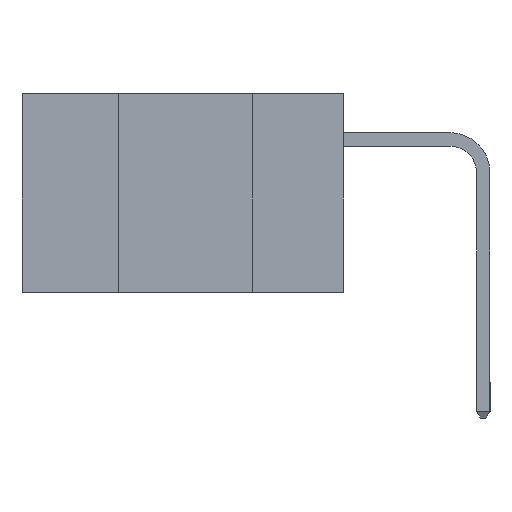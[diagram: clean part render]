
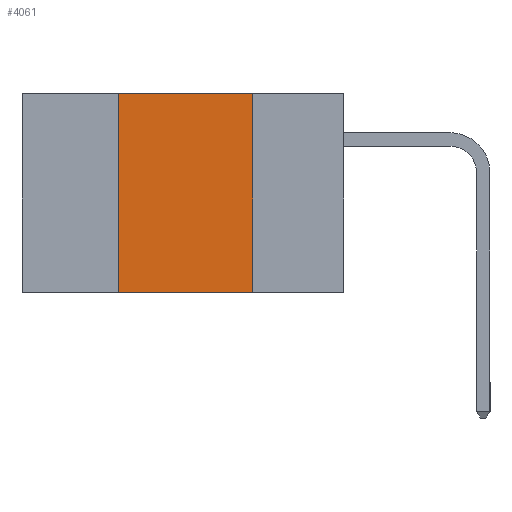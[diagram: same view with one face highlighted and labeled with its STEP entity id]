
A CAD part, left-side view. The second image highlights one B-rep face of the part: STEP entity #4061.
In plain terms, the highlighted planar face has unit normal (-1, 0, 0).
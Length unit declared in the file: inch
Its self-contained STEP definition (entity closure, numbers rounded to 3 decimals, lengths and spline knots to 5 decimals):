
#245 = CARTESIAN_POINT ( 'NONE',  ( 0., 0.17, -0.37 ) ) ;
#361 = CARTESIAN_POINT ( 'NONE',  ( 0., 0.6, -0.37 ) ) ;
#734 = CARTESIAN_POINT ( 'NONE',  ( 0., 0.42, 0. ) ) ;
#907 = EDGE_CURVE ( 'NONE', #4238, #4752, #8898, .T. ) ;
#1112 = VECTOR ( 'NONE', #9313, 39.37008 ) ;
#1890 = CARTESIAN_POINT ( 'NONE',  ( 0., 0.42, -0.37 ) ) ;
#2160 = VERTEX_POINT ( 'NONE', #245 ) ;
#2631 = CARTESIAN_POINT ( 'NONE',  ( 0., 0.6, 0. ) ) ;
#3139 = ORIENTED_EDGE ( 'NONE', *, *, #5192, .F. ) ;
#3257 = ORIENTED_EDGE ( 'NONE', *, *, #7800, .F. ) ;
#3527 = CARTESIAN_POINT ( 'NONE',  ( 0., 0.42, 0. ) ) ;
#3576 = PLANE ( 'NONE',  #9876 ) ;
#4061 = ADVANCED_FACE ( 'NONE', ( #12222 ), #3576, .F. ) ;
#4140 = DIRECTION ( 'NONE',  ( 0., -1., 0. ) ) ;
#4238 = VERTEX_POINT ( 'NONE', #1890 ) ;
#4752 = VERTEX_POINT ( 'NONE', #3527 ) ;
#5004 = CARTESIAN_POINT ( 'NONE',  ( 0., 0.17, 0. ) ) ;
#5192 = EDGE_CURVE ( 'NONE', #4752, #10579, #11038, .T. ) ;
#5395 = LINE ( 'NONE', #10466, #11558 ) ;
#5805 = CARTESIAN_POINT ( 'NONE',  ( 0., 0.6, 0. ) ) ;
#7460 = LINE ( 'NONE', #361, #1112 ) ;
#7720 = ORIENTED_EDGE ( 'NONE', *, *, #907, .F. ) ;
#7800 = EDGE_CURVE ( 'NONE', #10579, #2160, #5395, .T. ) ;
#8074 = DIRECTION ( 'NONE',  ( 0., 0., 1. ) ) ;
#8368 = EDGE_LOOP ( 'NONE', ( #3257, #3139, #7720, #9476 ) ) ;
#8457 = VECTOR ( 'NONE', #4140, 39.37008 ) ;
#8898 = LINE ( 'NONE', #734, #14234 ) ;
#9313 = DIRECTION ( 'NONE',  ( 0., -1., 0. ) ) ;
#9476 = ORIENTED_EDGE ( 'NONE', *, *, #12301, .T. ) ;
#9876 = AXIS2_PLACEMENT_3D ( 'NONE', #2631, #11264, #13079 ) ;
#10466 = CARTESIAN_POINT ( 'NONE',  ( 0., 0.17, 0. ) ) ;
#10579 = VERTEX_POINT ( 'NONE', #5004 ) ;
#11038 = LINE ( 'NONE', #5805, #8457 ) ;
#11264 = DIRECTION ( 'NONE',  ( 1., 0., 0. ) ) ;
#11558 = VECTOR ( 'NONE', #12419, 39.37008 ) ;
#12222 = FACE_OUTER_BOUND ( 'NONE', #8368, .T. ) ;
#12301 = EDGE_CURVE ( 'NONE', #4238, #2160, #7460, .T. ) ;
#12419 = DIRECTION ( 'NONE',  ( 0., 0., -1. ) ) ;
#13079 = DIRECTION ( 'NONE',  ( 0., 0., -1. ) ) ;
#14234 = VECTOR ( 'NONE', #8074, 39.37008 ) ;
